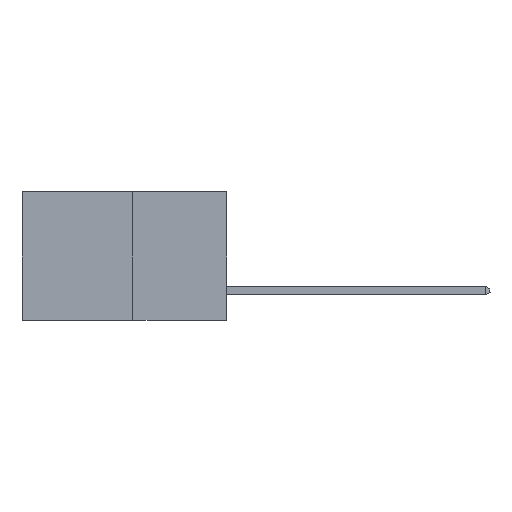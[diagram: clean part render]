
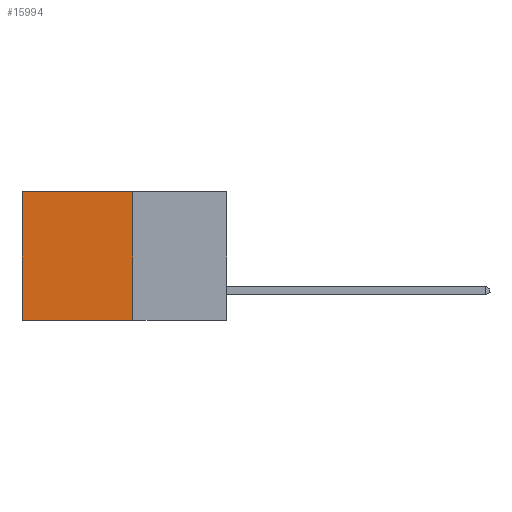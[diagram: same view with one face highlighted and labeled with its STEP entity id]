
A CAD part, left-side view. The second image highlights one B-rep face of the part: STEP entity #15994.
In plain terms, the highlighted planar face has unit normal (-1, 0, 0).
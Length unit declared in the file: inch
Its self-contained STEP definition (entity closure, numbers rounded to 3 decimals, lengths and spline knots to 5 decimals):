
#198 = DIRECTION ( 'NONE',  ( 0., 0., -1. ) ) ;
#477 = ORIENTED_EDGE ( 'NONE', *, *, #9405, .T. ) ;
#999 = CARTESIAN_POINT ( 'NONE',  ( 0.277, 0.27, -0.37 ) ) ;
#1097 = ORIENTED_EDGE ( 'NONE', *, *, #16463, .F. ) ;
#1124 = VERTEX_POINT ( 'NONE', #7032 ) ;
#2308 = ORIENTED_EDGE ( 'NONE', *, *, #16721, .F. ) ;
#2379 = DIRECTION ( 'NONE',  ( 0., 1., 0. ) ) ;
#2976 = VERTEX_POINT ( 'NONE', #7934 ) ;
#3284 = VECTOR ( 'NONE', #13936, 39.37008 ) ;
#4338 = CARTESIAN_POINT ( 'NONE',  ( 0.277, 0.59, 0. ) ) ;
#4363 = LINE ( 'NONE', #14508, #6960 ) ;
#4480 = AXIS2_PLACEMENT_3D ( 'NONE', #10553, #15700, #8004 ) ;
#4922 = CARTESIAN_POINT ( 'NONE',  ( 0.277, 0.59, -0.37 ) ) ;
#5301 = VERTEX_POINT ( 'NONE', #4338 ) ;
#5426 = PLANE ( 'NONE',  #4480 ) ;
#5818 = ORIENTED_EDGE ( 'NONE', *, *, #11309, .T. ) ;
#6960 = VECTOR ( 'NONE', #198, 39.37008 ) ;
#7032 = CARTESIAN_POINT ( 'NONE',  ( 0.277, 0.59, -0.37 ) ) ;
#7587 = VECTOR ( 'NONE', #2379, 39.37008 ) ;
#7934 = CARTESIAN_POINT ( 'NONE',  ( 0.277, 0.27, 0. ) ) ;
#8004 = DIRECTION ( 'NONE',  ( 0., 0., -1. ) ) ;
#8104 = LINE ( 'NONE', #9829, #14141 ) ;
#8661 = EDGE_LOOP ( 'NONE', ( #477, #1097, #2308, #5818 ) ) ;
#9405 = EDGE_CURVE ( 'NONE', #5301, #1124, #16612, .T. ) ;
#9829 = CARTESIAN_POINT ( 'NONE',  ( 0.277, 0.27, 0. ) ) ;
#10046 = VERTEX_POINT ( 'NONE', #13817 ) ;
#10553 = CARTESIAN_POINT ( 'NONE',  ( 0.277, 0.27, -0.37 ) ) ;
#11228 = DIRECTION ( 'NONE',  ( 0., 1., 0. ) ) ;
#11309 = EDGE_CURVE ( 'NONE', #2976, #5301, #8104, .T. ) ;
#11490 = FACE_OUTER_BOUND ( 'NONE', #8661, .T. ) ;
#13817 = CARTESIAN_POINT ( 'NONE',  ( 0.277, 0.27, -0.37 ) ) ;
#13936 = DIRECTION ( 'NONE',  ( 0., 0., -1. ) ) ;
#14141 = VECTOR ( 'NONE', #11228, 39.37008 ) ;
#14508 = CARTESIAN_POINT ( 'NONE',  ( 0.277, 0.27, -0.37 ) ) ;
#14841 = LINE ( 'NONE', #999, #7587 ) ;
#15700 = DIRECTION ( 'NONE',  ( 1., 0., 0. ) ) ;
#15994 = ADVANCED_FACE ( 'NONE', ( #11490 ), #5426, .F. ) ;
#16463 = EDGE_CURVE ( 'NONE', #10046, #1124, #14841, .T. ) ;
#16612 = LINE ( 'NONE', #4922, #3284 ) ;
#16721 = EDGE_CURVE ( 'NONE', #2976, #10046, #4363, .T. ) ;
